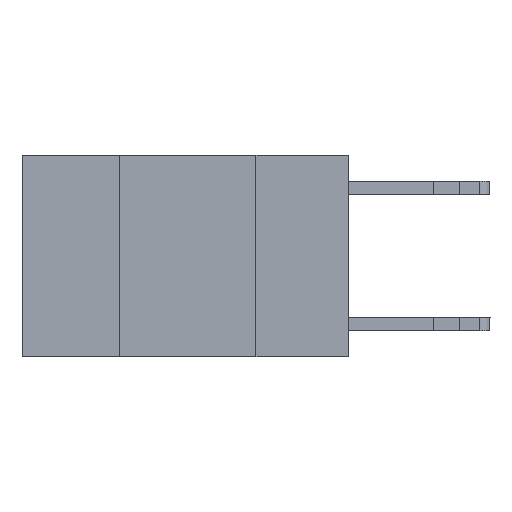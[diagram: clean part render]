
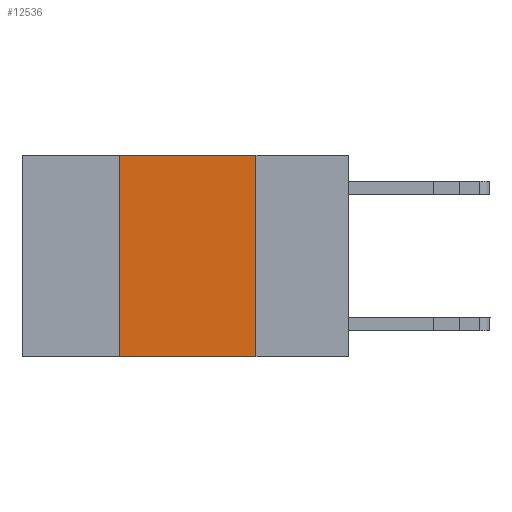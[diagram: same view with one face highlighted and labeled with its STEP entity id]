
A CAD part, left-side view. The second image highlights one B-rep face of the part: STEP entity #12536.
In plain terms, the highlighted planar face has unit normal (-1, 0, 0).
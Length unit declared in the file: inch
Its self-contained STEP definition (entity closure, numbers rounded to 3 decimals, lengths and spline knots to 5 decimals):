
#1 = VERTEX_POINT ( 'NONE', #3836 ) ;
#15 = LINE ( 'NONE', #13970, #7202 ) ;
#491 = CARTESIAN_POINT ( 'NONE',  ( 0., 0.17, 0. ) ) ;
#706 = DIRECTION ( 'NONE',  ( 1., 0., 0. ) ) ;
#2103 = LINE ( 'NONE', #491, #14846 ) ;
#2522 = DIRECTION ( 'NONE',  ( 0., -1., 0. ) ) ;
#2605 = CARTESIAN_POINT ( 'NONE',  ( 0., 0.17, 0. ) ) ;
#2827 = DIRECTION ( 'NONE',  ( 0., -1., 0. ) ) ;
#2975 = ORIENTED_EDGE ( 'NONE', *, *, #10846, .T. ) ;
#3114 = ORIENTED_EDGE ( 'NONE', *, *, #14658, .F. ) ;
#3623 = AXIS2_PLACEMENT_3D ( 'NONE', #11952, #706, #9525 ) ;
#3836 = CARTESIAN_POINT ( 'NONE',  ( 0., 0.17, -0.37 ) ) ;
#5151 = EDGE_LOOP ( 'NONE', ( #5227, #3114, #9078, #2975 ) ) ;
#5227 = ORIENTED_EDGE ( 'NONE', *, *, #14070, .F. ) ;
#6924 = CARTESIAN_POINT ( 'NONE',  ( 0., 0.42, 0. ) ) ;
#7202 = VECTOR ( 'NONE', #2827, 39.37008 ) ;
#7494 = FACE_OUTER_BOUND ( 'NONE', #5151, .T. ) ;
#8177 = DIRECTION ( 'NONE',  ( 0., 0., 1. ) ) ;
#9078 = ORIENTED_EDGE ( 'NONE', *, *, #12486, .F. ) ;
#9525 = DIRECTION ( 'NONE',  ( 0., 0., -1. ) ) ;
#10817 = CARTESIAN_POINT ( 'NONE',  ( 0., 0.42, -0.37 ) ) ;
#10846 = EDGE_CURVE ( 'NONE', #12579, #1, #15743, .T. ) ;
#11166 = VECTOR ( 'NONE', #8177, 39.37008 ) ;
#11271 = CARTESIAN_POINT ( 'NONE',  ( 0., 0.42, 0. ) ) ;
#11952 = CARTESIAN_POINT ( 'NONE',  ( 0., 0.6, 0. ) ) ;
#12164 = VERTEX_POINT ( 'NONE', #2605 ) ;
#12486 = EDGE_CURVE ( 'NONE', #12579, #15813, #14354, .T. ) ;
#12536 = ADVANCED_FACE ( 'NONE', ( #7494 ), #14337, .F. ) ;
#12556 = VECTOR ( 'NONE', #2522, 39.37008 ) ;
#12579 = VERTEX_POINT ( 'NONE', #10817 ) ;
#12985 = DIRECTION ( 'NONE',  ( 0., 0., -1. ) ) ;
#13611 = CARTESIAN_POINT ( 'NONE',  ( 0., 0.6, -0.37 ) ) ;
#13970 = CARTESIAN_POINT ( 'NONE',  ( 0., 0.6, 0. ) ) ;
#14070 = EDGE_CURVE ( 'NONE', #12164, #1, #2103, .T. ) ;
#14337 = PLANE ( 'NONE',  #3623 ) ;
#14354 = LINE ( 'NONE', #6924, #11166 ) ;
#14658 = EDGE_CURVE ( 'NONE', #15813, #12164, #15, .T. ) ;
#14846 = VECTOR ( 'NONE', #12985, 39.37008 ) ;
#15743 = LINE ( 'NONE', #13611, #12556 ) ;
#15813 = VERTEX_POINT ( 'NONE', #11271 ) ;
